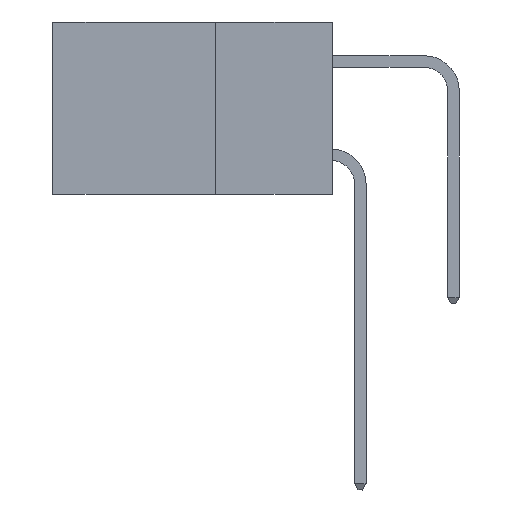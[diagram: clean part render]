
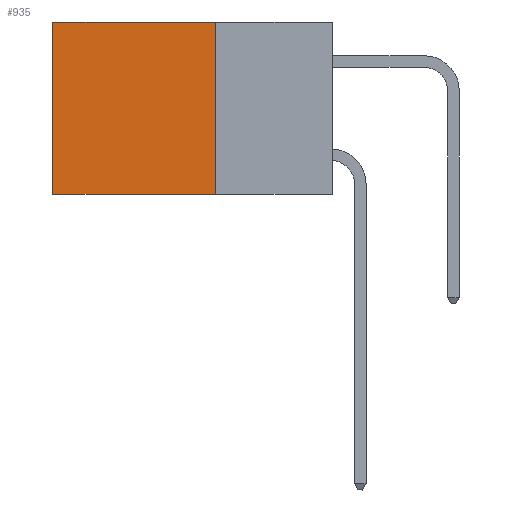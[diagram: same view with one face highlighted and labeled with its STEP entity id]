
A CAD part, left-side view. The second image highlights one B-rep face of the part: STEP entity #935.
In plain terms, the highlighted planar face has unit normal (-1, 0, 0).
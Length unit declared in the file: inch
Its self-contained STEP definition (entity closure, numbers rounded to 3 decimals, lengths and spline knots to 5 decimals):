
#80 = CARTESIAN_POINT ( 'NONE',  ( 0.298, 0.25, 0. ) ) ;
#645 = PLANE ( 'NONE',  #3817 ) ;
#935 = ADVANCED_FACE ( 'NONE', ( #5184 ), #645, .F. ) ;
#1184 = EDGE_CURVE ( 'NONE', #9631, #12302, #6363, .T. ) ;
#1314 = LINE ( 'NONE', #10880, #11495 ) ;
#1478 = CARTESIAN_POINT ( 'NONE',  ( 0.298, 0.25, 0. ) ) ;
#1497 = LINE ( 'NONE', #10521, #11840 ) ;
#1797 = ORIENTED_EDGE ( 'NONE', *, *, #11573, .T. ) ;
#2277 = CARTESIAN_POINT ( 'NONE',  ( 0.298, 0.25, -0.37 ) ) ;
#2828 = DIRECTION ( 'NONE',  ( 0., 0., -1. ) ) ;
#3507 = DIRECTION ( 'NONE',  ( 0., 0., -1. ) ) ;
#3748 = VERTEX_POINT ( 'NONE', #4996 ) ;
#3817 = AXIS2_PLACEMENT_3D ( 'NONE', #1478, #8356, #3507 ) ;
#3828 = VECTOR ( 'NONE', #6183, 39.37008 ) ;
#4996 = CARTESIAN_POINT ( 'NONE',  ( 0.298, 0.6, 0. ) ) ;
#5081 = ORIENTED_EDGE ( 'NONE', *, *, #10695, .T. ) ;
#5184 = FACE_OUTER_BOUND ( 'NONE', #7920, .T. ) ;
#5228 = VECTOR ( 'NONE', #11170, 39.37008 ) ;
#6183 = DIRECTION ( 'NONE',  ( 0., 1., 0. ) ) ;
#6363 = LINE ( 'NONE', #2277, #3828 ) ;
#6644 = CARTESIAN_POINT ( 'NONE',  ( 0.298, 0.6, -0.37 ) ) ;
#6657 = ORIENTED_EDGE ( 'NONE', *, *, #1184, .F. ) ;
#7044 = DIRECTION ( 'NONE',  ( 0., 1., 0. ) ) ;
#7465 = LINE ( 'NONE', #10216, #5228 ) ;
#7920 = EDGE_LOOP ( 'NONE', ( #5081, #6657, #11896, #1797 ) ) ;
#8031 = CARTESIAN_POINT ( 'NONE',  ( 0.298, 0.25, -0.37 ) ) ;
#8356 = DIRECTION ( 'NONE',  ( 1., 0., 0. ) ) ;
#9631 = VERTEX_POINT ( 'NONE', #8031 ) ;
#10216 = CARTESIAN_POINT ( 'NONE',  ( 0.298, 0.25, 0. ) ) ;
#10521 = CARTESIAN_POINT ( 'NONE',  ( 0.298, 0.6, 0. ) ) ;
#10695 = EDGE_CURVE ( 'NONE', #3748, #12302, #1497, .T. ) ;
#10855 = VERTEX_POINT ( 'NONE', #80 ) ;
#10880 = CARTESIAN_POINT ( 'NONE',  ( 0.298, 0.25, 0. ) ) ;
#11170 = DIRECTION ( 'NONE',  ( 0., 0., -1. ) ) ;
#11232 = EDGE_CURVE ( 'NONE', #10855, #9631, #7465, .T. ) ;
#11495 = VECTOR ( 'NONE', #7044, 39.37008 ) ;
#11573 = EDGE_CURVE ( 'NONE', #10855, #3748, #1314, .T. ) ;
#11840 = VECTOR ( 'NONE', #2828, 39.37008 ) ;
#11896 = ORIENTED_EDGE ( 'NONE', *, *, #11232, .F. ) ;
#12302 = VERTEX_POINT ( 'NONE', #6644 ) ;
